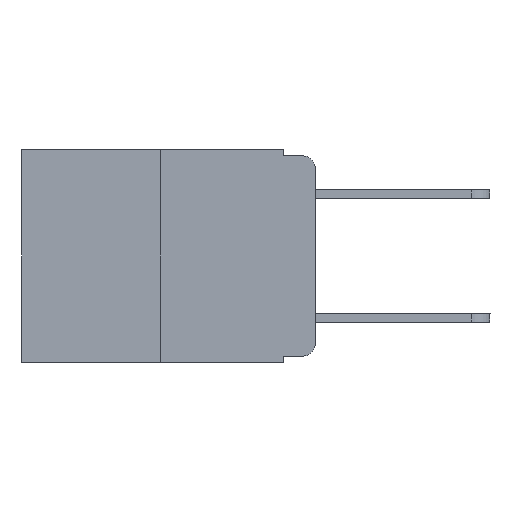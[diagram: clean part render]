
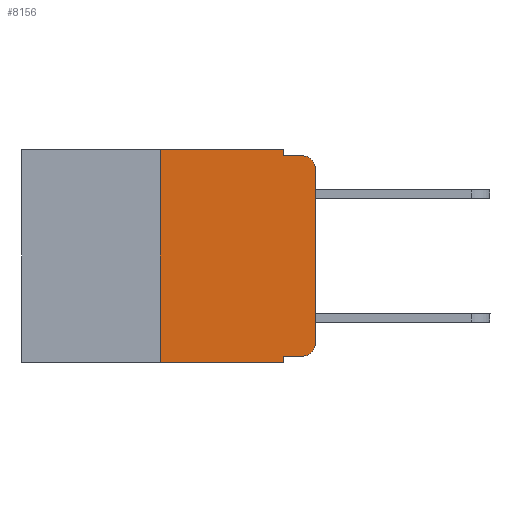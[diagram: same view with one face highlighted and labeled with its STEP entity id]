
A CAD part, left-side view. The second image highlights one B-rep face of the part: STEP entity #8156.
In plain terms, the highlighted planar face has unit normal (-1, 0, 0).
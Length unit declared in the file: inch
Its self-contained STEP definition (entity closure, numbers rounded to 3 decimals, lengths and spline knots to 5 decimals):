
#360 = LINE ( 'NONE', #15809, #4962 ) ;
#400 = VECTOR ( 'NONE', #10891, 39.37008 ) ;
#435 = CARTESIAN_POINT ( 'NONE',  ( 0., 0.051, 0. ) ) ;
#602 = DIRECTION ( 'NONE',  ( 0., 0., -1. ) ) ;
#658 = ORIENTED_EDGE ( 'NONE', *, *, #9127, .T. ) ;
#741 = DIRECTION ( 'NONE',  ( 1., 0., 0. ) ) ;
#911 = AXIS2_PLACEMENT_3D ( 'NONE', #10037, #741, #16379 ) ;
#927 = CARTESIAN_POINT ( 'NONE',  ( 0., 0., -0.03 ) ) ;
#1153 = EDGE_CURVE ( 'NONE', #3874, #8249, #10920, .T. ) ;
#1797 = DIRECTION ( 'NONE',  ( 0., 0., -1. ) ) ;
#1830 = ORIENTED_EDGE ( 'NONE', *, *, #5041, .T. ) ;
#1864 = ORIENTED_EDGE ( 'NONE', *, *, #8315, .F. ) ;
#1997 = ORIENTED_EDGE ( 'NONE', *, *, #19584, .F. ) ;
#2053 = EDGE_CURVE ( 'NONE', #18226, #3874, #12601, .T. ) ;
#2229 = VERTEX_POINT ( 'NONE', #19414 ) ;
#2730 = CARTESIAN_POINT ( 'NONE',  ( 0., 0.02, -0.333 ) ) ;
#2840 = FACE_OUTER_BOUND ( 'NONE', #16310, .T. ) ;
#2934 = ORIENTED_EDGE ( 'NONE', *, *, #2053, .T. ) ;
#3718 = VERTEX_POINT ( 'NONE', #17168 ) ;
#3874 = VERTEX_POINT ( 'NONE', #927 ) ;
#3893 = PLANE ( 'NONE',  #911 ) ;
#4576 = DIRECTION ( 'NONE',  ( 0., 0., -1. ) ) ;
#4695 = DIRECTION ( 'NONE',  ( 0., -1., 0. ) ) ;
#4962 = VECTOR ( 'NONE', #4695, 39.37008 ) ;
#5041 = EDGE_CURVE ( 'NONE', #17870, #18226, #6982, .T. ) ;
#5328 = CARTESIAN_POINT ( 'NONE',  ( 0., 0.02, -0.03 ) ) ;
#5809 = DIRECTION ( 'NONE',  ( 0., -1., 0. ) ) ;
#6242 = EDGE_CURVE ( 'NONE', #2229, #8249, #7473, .T. ) ;
#6649 = DIRECTION ( 'NONE',  ( 0., 0., 1. ) ) ;
#6683 = LINE ( 'NONE', #18723, #400 ) ;
#6982 = CIRCLE ( 'NONE', #16646, 0.02 ) ;
#7473 = LINE ( 'NONE', #9954, #15548 ) ;
#8156 = ADVANCED_FACE ( 'NONE', ( #2840 ), #3893, .F. ) ;
#8249 = VERTEX_POINT ( 'NONE', #16575 ) ;
#8315 = EDGE_CURVE ( 'NONE', #19609, #8776, #6683, .T. ) ;
#8509 = DIRECTION ( 'NONE',  ( 0., -1., 0. ) ) ;
#8776 = VERTEX_POINT ( 'NONE', #19913 ) ;
#9110 = LINE ( 'NONE', #19714, #10814 ) ;
#9127 = EDGE_CURVE ( 'NONE', #11769, #17870, #11566, .T. ) ;
#9201 = VECTOR ( 'NONE', #6649, 39.37008 ) ;
#9863 = LINE ( 'NONE', #12211, #17921 ) ;
#9948 = DIRECTION ( 'NONE',  ( 0., 0., -1. ) ) ;
#9954 = CARTESIAN_POINT ( 'NONE',  ( 0., 0.051, -0.01 ) ) ;
#10037 = CARTESIAN_POINT ( 'NONE',  ( 0., 0.473, 0. ) ) ;
#10097 = CARTESIAN_POINT ( 'NONE',  ( 0., 0.02, -0.313 ) ) ;
#10544 = CARTESIAN_POINT ( 'NONE',  ( 0., 0., -0.313 ) ) ;
#10814 = VECTOR ( 'NONE', #5809, 39.37008 ) ;
#10891 = DIRECTION ( 'NONE',  ( 0., 0., 1. ) ) ;
#10920 = CIRCLE ( 'NONE', #20079, 0.02 ) ;
#11566 = LINE ( 'NONE', #17705, #18375 ) ;
#11663 = DIRECTION ( 'NONE',  ( -1., 0., 0. ) ) ;
#11712 = CARTESIAN_POINT ( 'NONE',  ( 0., 0.051, -0.333 ) ) ;
#11769 = VERTEX_POINT ( 'NONE', #11712 ) ;
#12211 = CARTESIAN_POINT ( 'NONE',  ( 0., 0.051, 0. ) ) ;
#12238 = EDGE_CURVE ( 'NONE', #8776, #3718, #9110, .T. ) ;
#12601 = LINE ( 'NONE', #16021, #9201 ) ;
#12654 = CARTESIAN_POINT ( 'NONE',  ( 0., 0.25, -0.343 ) ) ;
#13928 = ORIENTED_EDGE ( 'NONE', *, *, #12238, .F. ) ;
#14723 = DIRECTION ( 'NONE',  ( 0., -1., 0. ) ) ;
#14875 = VECTOR ( 'NONE', #1797, 39.37008 ) ;
#15167 = ORIENTED_EDGE ( 'NONE', *, *, #6242, .F. ) ;
#15548 = VECTOR ( 'NONE', #8509, 39.37008 ) ;
#15572 = EDGE_CURVE ( 'NONE', #3718, #2229, #9863, .T. ) ;
#15809 = CARTESIAN_POINT ( 'NONE',  ( 0., 0.473, -0.343 ) ) ;
#16021 = CARTESIAN_POINT ( 'NONE',  ( 0., 0., 0. ) ) ;
#16161 = EDGE_CURVE ( 'NONE', #19609, #16603, #360, .T. ) ;
#16212 = ORIENTED_EDGE ( 'NONE', *, *, #16161, .T. ) ;
#16310 = EDGE_LOOP ( 'NONE', ( #2934, #17349, #15167, #18102, #13928, #1864, #16212, #1997, #658, #1830 ) ) ;
#16379 = DIRECTION ( 'NONE',  ( 0., 0., -1. ) ) ;
#16575 = CARTESIAN_POINT ( 'NONE',  ( 0., 0.02, -0.01 ) ) ;
#16603 = VERTEX_POINT ( 'NONE', #18047 ) ;
#16646 = AXIS2_PLACEMENT_3D ( 'NONE', #10097, #11663, #9948 ) ;
#17168 = CARTESIAN_POINT ( 'NONE',  ( 0., 0.051, 0. ) ) ;
#17349 = ORIENTED_EDGE ( 'NONE', *, *, #1153, .T. ) ;
#17705 = CARTESIAN_POINT ( 'NONE',  ( 0., 0.051, -0.333 ) ) ;
#17799 = DIRECTION ( 'NONE',  ( -1., 0., 0. ) ) ;
#17870 = VERTEX_POINT ( 'NONE', #2730 ) ;
#17921 = VECTOR ( 'NONE', #4576, 39.37008 ) ;
#18019 = LINE ( 'NONE', #435, #14875 ) ;
#18047 = CARTESIAN_POINT ( 'NONE',  ( 0., 0.051, -0.343 ) ) ;
#18102 = ORIENTED_EDGE ( 'NONE', *, *, #15572, .F. ) ;
#18226 = VERTEX_POINT ( 'NONE', #10544 ) ;
#18375 = VECTOR ( 'NONE', #14723, 39.37008 ) ;
#18723 = CARTESIAN_POINT ( 'NONE',  ( 0., 0.25, 0. ) ) ;
#19414 = CARTESIAN_POINT ( 'NONE',  ( 0., 0.051, -0.01 ) ) ;
#19584 = EDGE_CURVE ( 'NONE', #11769, #16603, #18019, .T. ) ;
#19609 = VERTEX_POINT ( 'NONE', #12654 ) ;
#19714 = CARTESIAN_POINT ( 'NONE',  ( 0., 0.473, 0. ) ) ;
#19913 = CARTESIAN_POINT ( 'NONE',  ( 0., 0.25, 0. ) ) ;
#20079 = AXIS2_PLACEMENT_3D ( 'NONE', #5328, #17799, #602 ) ;
